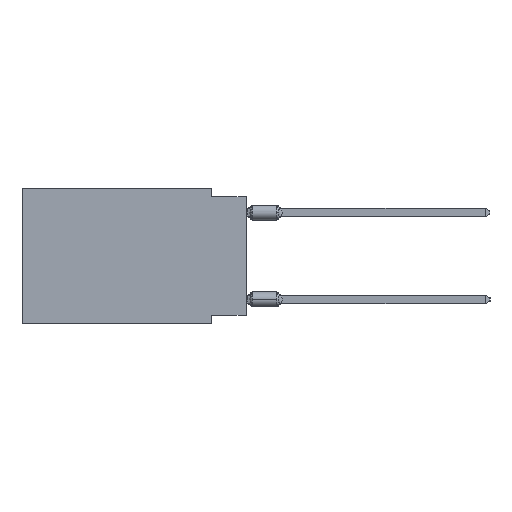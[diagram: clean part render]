
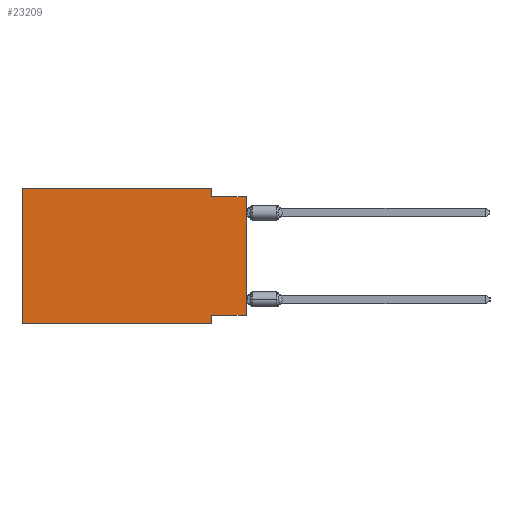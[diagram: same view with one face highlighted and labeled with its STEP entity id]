
A CAD part, left-side view. The second image highlights one B-rep face of the part: STEP entity #23209.
In plain terms, the highlighted planar face has unit normal (-1, 0, 0).
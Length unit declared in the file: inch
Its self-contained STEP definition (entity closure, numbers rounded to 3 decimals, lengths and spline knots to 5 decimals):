
#110 = VERTEX_POINT ( 'NONE', #44304 ) ;
#619 = LINE ( 'NONE', #57673, #19194 ) ;
#935 = EDGE_CURVE ( 'NONE', #5337, #39704, #619, .T. ) ;
#1160 = VECTOR ( 'NONE', #38731, 39.37008 ) ;
#2135 = CARTESIAN_POINT ( 'NONE',  ( 0., 0.645, 0. ) ) ;
#4151 = DIRECTION ( 'NONE',  ( 0., 0., -1. ) ) ;
#5337 = VERTEX_POINT ( 'NONE', #20401 ) ;
#6158 = DIRECTION ( 'NONE',  ( 0., -1., 0. ) ) ;
#6452 = CARTESIAN_POINT ( 'NONE',  ( 0., 0.645, 0. ) ) ;
#7457 = ORIENTED_EDGE ( 'NONE', *, *, #19064, .F. ) ;
#7503 = VERTEX_POINT ( 'NONE', #52335 ) ;
#7651 = VECTOR ( 'NONE', #58002, 39.37008 ) ;
#8276 = CARTESIAN_POINT ( 'NONE',  ( 0., 0.1, -0.39 ) ) ;
#13479 = PLANE ( 'NONE',  #57230 ) ;
#13742 = VECTOR ( 'NONE', #24231, 39.37008 ) ;
#14377 = FACE_OUTER_BOUND ( 'NONE', #33749, .T. ) ;
#14489 = ORIENTED_EDGE ( 'NONE', *, *, #21326, .F. ) ;
#15101 = CARTESIAN_POINT ( 'NONE',  ( 0., 0.1, -0.39 ) ) ;
#19064 = EDGE_CURVE ( 'NONE', #5337, #25911, #56445, .T. ) ;
#19194 = VECTOR ( 'NONE', #19656, 39.37008 ) ;
#19296 = DIRECTION ( 'NONE',  ( 0., 0., -1. ) ) ;
#19631 = CARTESIAN_POINT ( 'NONE',  ( 0., 0.1, -0.025 ) ) ;
#19656 = DIRECTION ( 'NONE',  ( 0., 0., 1. ) ) ;
#20401 = CARTESIAN_POINT ( 'NONE',  ( 0., 0., -0.365 ) ) ;
#20831 = DIRECTION ( 'NONE',  ( 0., -1., 0. ) ) ;
#21169 = LINE ( 'NONE', #6452, #7651 ) ;
#21326 = EDGE_CURVE ( 'NONE', #25911, #26088, #23430, .T. ) ;
#22476 = CARTESIAN_POINT ( 'NONE',  ( 0., 0.645, 0. ) ) ;
#22870 = CARTESIAN_POINT ( 'NONE',  ( 0., 0.1, 0. ) ) ;
#23069 = DIRECTION ( 'NONE',  ( 0., -1., 0. ) ) ;
#23209 = ADVANCED_FACE ( 'NONE', ( #14377 ), #13479, .F. ) ;
#23314 = CARTESIAN_POINT ( 'NONE',  ( 0., 0., -0.025 ) ) ;
#23430 = LINE ( 'NONE', #15101, #1160 ) ;
#24231 = DIRECTION ( 'NONE',  ( 0., 1., 0. ) ) ;
#25440 = LINE ( 'NONE', #44158, #30309 ) ;
#25568 = EDGE_CURVE ( 'NONE', #31556, #7503, #31667, .T. ) ;
#25911 = VERTEX_POINT ( 'NONE', #43588 ) ;
#25979 = EDGE_CURVE ( 'NONE', #110, #31556, #21169, .T. ) ;
#26088 = VERTEX_POINT ( 'NONE', #8276 ) ;
#26254 = ORIENTED_EDGE ( 'NONE', *, *, #25979, .F. ) ;
#28498 = CARTESIAN_POINT ( 'NONE',  ( 0., 0.645, 0. ) ) ;
#30309 = VECTOR ( 'NONE', #20831, 39.37008 ) ;
#31556 = VERTEX_POINT ( 'NONE', #2135 ) ;
#31667 = LINE ( 'NONE', #22476, #35070 ) ;
#31760 = ORIENTED_EDGE ( 'NONE', *, *, #51549, .T. ) ;
#33749 = EDGE_LOOP ( 'NONE', ( #52484, #49196, #34732, #48090, #26254, #31760, #14489, #7457 ) ) ;
#34732 = ORIENTED_EDGE ( 'NONE', *, *, #49351, .F. ) ;
#35070 = VECTOR ( 'NONE', #23069, 39.37008 ) ;
#38731 = DIRECTION ( 'NONE',  ( 0., 0., -1. ) ) ;
#39704 = VERTEX_POINT ( 'NONE', #23314 ) ;
#42305 = DIRECTION ( 'NONE',  ( 1., 0., 0. ) ) ;
#43510 = VECTOR ( 'NONE', #6158, 39.37008 ) ;
#43588 = CARTESIAN_POINT ( 'NONE',  ( 0., 0.1, -0.365 ) ) ;
#44158 = CARTESIAN_POINT ( 'NONE',  ( 0., 0., -0.025 ) ) ;
#44205 = CARTESIAN_POINT ( 'NONE',  ( 0., 0.645, -0.39 ) ) ;
#44304 = CARTESIAN_POINT ( 'NONE',  ( 0., 0.645, -0.39 ) ) ;
#44934 = VECTOR ( 'NONE', #4151, 39.37008 ) ;
#47843 = CARTESIAN_POINT ( 'NONE',  ( 0., 0., -0.365 ) ) ;
#48090 = ORIENTED_EDGE ( 'NONE', *, *, #25568, .F. ) ;
#49196 = ORIENTED_EDGE ( 'NONE', *, *, #50117, .F. ) ;
#49351 = EDGE_CURVE ( 'NONE', #7503, #55655, #59365, .T. ) ;
#50117 = EDGE_CURVE ( 'NONE', #55655, #39704, #25440, .T. ) ;
#51549 = EDGE_CURVE ( 'NONE', #110, #26088, #53100, .T. ) ;
#52335 = CARTESIAN_POINT ( 'NONE',  ( 0., 0.1, 0. ) ) ;
#52484 = ORIENTED_EDGE ( 'NONE', *, *, #935, .T. ) ;
#53100 = LINE ( 'NONE', #44205, #43510 ) ;
#55655 = VERTEX_POINT ( 'NONE', #19631 ) ;
#56445 = LINE ( 'NONE', #47843, #13742 ) ;
#57230 = AXIS2_PLACEMENT_3D ( 'NONE', #28498, #42305, #19296 ) ;
#57673 = CARTESIAN_POINT ( 'NONE',  ( 0., 0., 0. ) ) ;
#58002 = DIRECTION ( 'NONE',  ( 0., 0., 1. ) ) ;
#59365 = LINE ( 'NONE', #22870, #44934 ) ;
